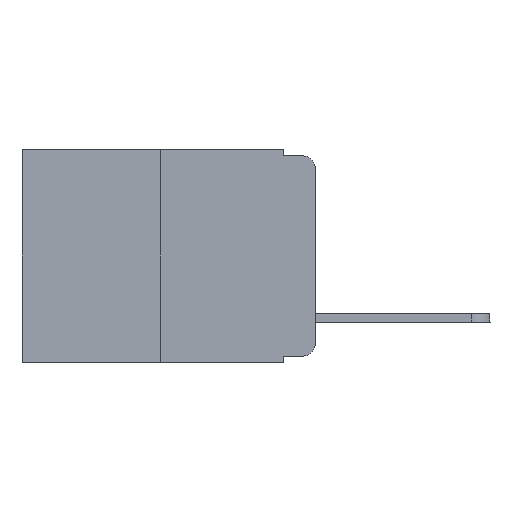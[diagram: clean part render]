
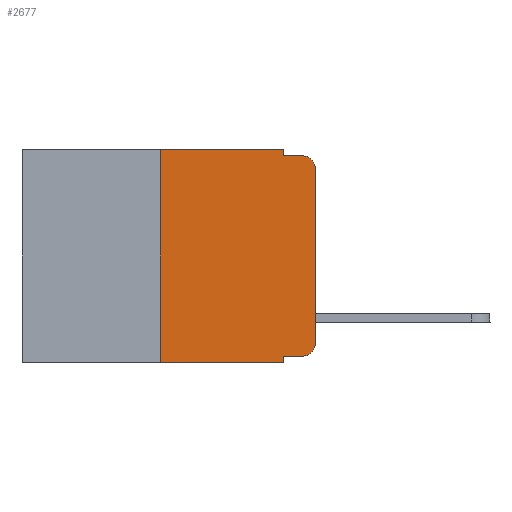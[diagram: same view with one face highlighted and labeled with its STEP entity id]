
A CAD part, left-side view. The second image highlights one B-rep face of the part: STEP entity #2677.
In plain terms, the highlighted planar face has unit normal (-1, 0, 0).
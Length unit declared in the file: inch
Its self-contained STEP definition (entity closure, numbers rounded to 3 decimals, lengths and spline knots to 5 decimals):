
#48 = CARTESIAN_POINT ( 'NONE',  ( 0., 0.051, -0.01 ) ) ;
#63 = VERTEX_POINT ( 'NONE', #10803 ) ;
#186 = VECTOR ( 'NONE', #12061, 39.37008 ) ;
#195 = EDGE_CURVE ( 'NONE', #1609, #7321, #6011, .T. ) ;
#367 = DIRECTION ( 'NONE',  ( 0., -1., 0. ) ) ;
#579 = EDGE_LOOP ( 'NONE', ( #2813, #5245, #6647, #13852, #12704, #3955, #4659, #11346, #15004, #2516 ) ) ;
#1119 = LINE ( 'NONE', #13410, #9143 ) ;
#1134 = DIRECTION ( 'NONE',  ( 0., 0., -1. ) ) ;
#1341 = VERTEX_POINT ( 'NONE', #6375 ) ;
#1522 = VERTEX_POINT ( 'NONE', #6757 ) ;
#1530 = VERTEX_POINT ( 'NONE', #7869 ) ;
#1609 = VERTEX_POINT ( 'NONE', #15646 ) ;
#1704 = CARTESIAN_POINT ( 'NONE',  ( 0., 0.25, 0. ) ) ;
#2069 = LINE ( 'NONE', #11604, #7953 ) ;
#2124 = DIRECTION ( 'NONE',  ( -1., 0., 0. ) ) ;
#2189 = CARTESIAN_POINT ( 'NONE',  ( 0., 0.25, -0.343 ) ) ;
#2266 = EDGE_CURVE ( 'NONE', #1341, #1530, #11203, .T. ) ;
#2295 = EDGE_CURVE ( 'NONE', #63, #1609, #13724, .T. ) ;
#2516 = ORIENTED_EDGE ( 'NONE', *, *, #195, .T. ) ;
#2661 = DIRECTION ( 'NONE',  ( 0., 0., 1. ) ) ;
#2677 = ADVANCED_FACE ( 'NONE', ( #14093 ), #15966, .F. ) ;
#2813 = ORIENTED_EDGE ( 'NONE', *, *, #15596, .T. ) ;
#2984 = VERTEX_POINT ( 'NONE', #2189 ) ;
#3647 = VERTEX_POINT ( 'NONE', #12409 ) ;
#3758 = CARTESIAN_POINT ( 'NONE',  ( 0., 0.051, 0. ) ) ;
#3955 = ORIENTED_EDGE ( 'NONE', *, *, #10832, .F. ) ;
#4659 = ORIENTED_EDGE ( 'NONE', *, *, #7965, .T. ) ;
#4729 = LINE ( 'NONE', #10816, #186 ) ;
#5245 = ORIENTED_EDGE ( 'NONE', *, *, #2266, .T. ) ;
#5753 = VERTEX_POINT ( 'NONE', #48 ) ;
#5883 = VECTOR ( 'NONE', #8948, 39.37008 ) ;
#6011 = CIRCLE ( 'NONE', #13132, 0.02 ) ;
#6375 = CARTESIAN_POINT ( 'NONE',  ( 0., 0., -0.03 ) ) ;
#6647 = ORIENTED_EDGE ( 'NONE', *, *, #7268, .F. ) ;
#6757 = CARTESIAN_POINT ( 'NONE',  ( 0., 0.051, -0.343 ) ) ;
#6817 = LINE ( 'NONE', #10145, #9379 ) ;
#7268 = EDGE_CURVE ( 'NONE', #5753, #1530, #13683, .T. ) ;
#7321 = VERTEX_POINT ( 'NONE', #12824 ) ;
#7326 = CARTESIAN_POINT ( 'NONE',  ( 0., 0.473, 0. ) ) ;
#7645 = AXIS2_PLACEMENT_3D ( 'NONE', #12629, #9025, #13953 ) ;
#7869 = CARTESIAN_POINT ( 'NONE',  ( 0., 0.02, -0.01 ) ) ;
#7953 = VECTOR ( 'NONE', #9300, 39.37008 ) ;
#7965 = EDGE_CURVE ( 'NONE', #2984, #1522, #4729, .T. ) ;
#8419 = CARTESIAN_POINT ( 'NONE',  ( 0., 0.02, -0.313 ) ) ;
#8580 = DIRECTION ( 'NONE',  ( 1., 0., 0. ) ) ;
#8617 = LINE ( 'NONE', #13347, #10734 ) ;
#8948 = DIRECTION ( 'NONE',  ( 0., -1., 0. ) ) ;
#9025 = DIRECTION ( 'NONE',  ( -1., 0., 0. ) ) ;
#9078 = VECTOR ( 'NONE', #367, 39.37008 ) ;
#9143 = VECTOR ( 'NONE', #14634, 39.37008 ) ;
#9300 = DIRECTION ( 'NONE',  ( 0., 0., -1. ) ) ;
#9377 = EDGE_CURVE ( 'NONE', #3647, #5753, #9733, .T. ) ;
#9379 = VECTOR ( 'NONE', #2661, 39.37008 ) ;
#9686 = DIRECTION ( 'NONE',  ( 0., 0., -1. ) ) ;
#9733 = LINE ( 'NONE', #3758, #15568 ) ;
#10144 = EDGE_CURVE ( 'NONE', #63, #1522, #2069, .T. ) ;
#10145 = CARTESIAN_POINT ( 'NONE',  ( 0., 0., 0. ) ) ;
#10734 = VECTOR ( 'NONE', #10982, 39.37008 ) ;
#10803 = CARTESIAN_POINT ( 'NONE',  ( 0., 0.051, -0.333 ) ) ;
#10816 = CARTESIAN_POINT ( 'NONE',  ( 0., 0.473, -0.343 ) ) ;
#10832 = EDGE_CURVE ( 'NONE', #2984, #14475, #1119, .T. ) ;
#10982 = DIRECTION ( 'NONE',  ( 0., -1., 0. ) ) ;
#11203 = CIRCLE ( 'NONE', #7645, 0.02 ) ;
#11278 = AXIS2_PLACEMENT_3D ( 'NONE', #7326, #8580, #1134 ) ;
#11346 = ORIENTED_EDGE ( 'NONE', *, *, #10144, .F. ) ;
#11604 = CARTESIAN_POINT ( 'NONE',  ( 0., 0.051, 0. ) ) ;
#12061 = DIRECTION ( 'NONE',  ( 0., -1., 0. ) ) ;
#12409 = CARTESIAN_POINT ( 'NONE',  ( 0., 0.051, 0. ) ) ;
#12629 = CARTESIAN_POINT ( 'NONE',  ( 0., 0.02, -0.03 ) ) ;
#12704 = ORIENTED_EDGE ( 'NONE', *, *, #14759, .F. ) ;
#12824 = CARTESIAN_POINT ( 'NONE',  ( 0., 0., -0.313 ) ) ;
#13132 = AXIS2_PLACEMENT_3D ( 'NONE', #8419, #2124, #9686 ) ;
#13347 = CARTESIAN_POINT ( 'NONE',  ( 0., 0.473, 0. ) ) ;
#13410 = CARTESIAN_POINT ( 'NONE',  ( 0., 0.25, 0. ) ) ;
#13683 = LINE ( 'NONE', #15073, #5883 ) ;
#13723 = DIRECTION ( 'NONE',  ( 0., 0., -1. ) ) ;
#13724 = LINE ( 'NONE', #15200, #9078 ) ;
#13852 = ORIENTED_EDGE ( 'NONE', *, *, #9377, .F. ) ;
#13953 = DIRECTION ( 'NONE',  ( 0., 0., -1. ) ) ;
#14093 = FACE_OUTER_BOUND ( 'NONE', #579, .T. ) ;
#14475 = VERTEX_POINT ( 'NONE', #1704 ) ;
#14634 = DIRECTION ( 'NONE',  ( 0., 0., 1. ) ) ;
#14759 = EDGE_CURVE ( 'NONE', #14475, #3647, #8617, .T. ) ;
#15004 = ORIENTED_EDGE ( 'NONE', *, *, #2295, .T. ) ;
#15073 = CARTESIAN_POINT ( 'NONE',  ( 0., 0.051, -0.01 ) ) ;
#15200 = CARTESIAN_POINT ( 'NONE',  ( 0., 0.051, -0.333 ) ) ;
#15568 = VECTOR ( 'NONE', #13723, 39.37008 ) ;
#15596 = EDGE_CURVE ( 'NONE', #7321, #1341, #6817, .T. ) ;
#15646 = CARTESIAN_POINT ( 'NONE',  ( 0., 0.02, -0.333 ) ) ;
#15966 = PLANE ( 'NONE',  #11278 ) ;
